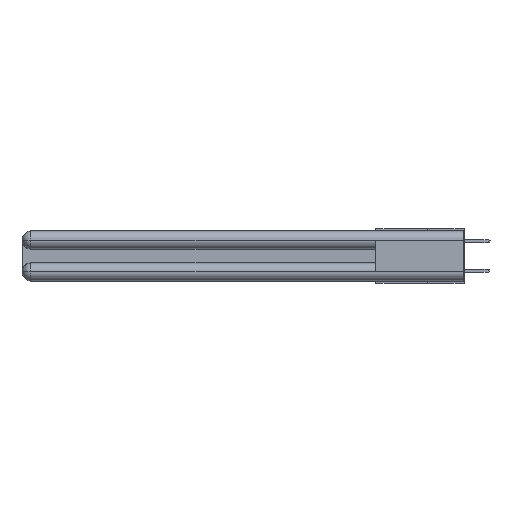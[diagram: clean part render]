
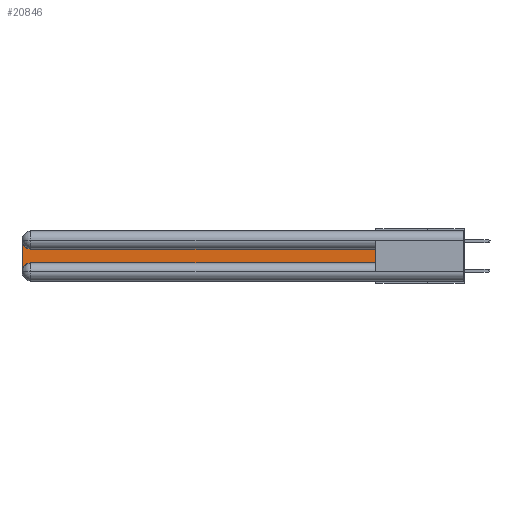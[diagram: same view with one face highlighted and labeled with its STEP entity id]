
A CAD part, left-side view. The second image highlights one B-rep face of the part: STEP entity #20846.
In plain terms, the highlighted planar face has unit normal (-1, 0, 0).
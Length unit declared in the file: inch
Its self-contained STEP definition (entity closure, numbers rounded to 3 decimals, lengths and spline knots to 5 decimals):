
#2008 = FACE_OUTER_BOUND ( 'NONE', #24947, .T. ) ;
#2785 = AXIS2_PLACEMENT_3D ( 'NONE', #3034, #21613, #30291 ) ;
#3034 = CARTESIAN_POINT ( 'NONE',  ( 0.075, 3., -0.1225 ) ) ;
#3149 = PLANE ( 'NONE',  #2785 ) ;
#3286 = EDGE_CURVE ( 'NONE', #6615, #20728, #32143, .T. ) ;
#3447 = VERTEX_POINT ( 'NONE', #4964 ) ;
#3922 = EDGE_CURVE ( 'NONE', #20071, #6615, #4162, .T. ) ;
#4162 = LINE ( 'NONE', #4510, #31746 ) ;
#4510 = CARTESIAN_POINT ( 'NONE',  ( 0.075, 3., -0.2175 ) ) ;
#4614 = DIRECTION ( 'NONE',  ( 0., 0., -1. ) ) ;
#4964 = CARTESIAN_POINT ( 'NONE',  ( 0.075, 0.6, -0.2175 ) ) ;
#6251 = EDGE_CURVE ( 'NONE', #20728, #3447, #19456, .T. ) ;
#6615 = VERTEX_POINT ( 'NONE', #19800 ) ;
#10061 = VERTEX_POINT ( 'NONE', #17948 ) ;
#10757 = VECTOR ( 'NONE', #32738, 39.37008 ) ;
#11026 = CARTESIAN_POINT ( 'NONE',  ( 0.075, 2.94, -0.0625 ) ) ;
#11785 = ORIENTED_EDGE ( 'NONE', *, *, #22195, .T. ) ;
#11967 = EDGE_CURVE ( 'NONE', #10061, #21042, #24591, .T. ) ;
#12924 = DIRECTION ( 'NONE',  ( 0., -1., 0. ) ) ;
#13314 = VECTOR ( 'NONE', #24391, 39.37008 ) ;
#14366 = ORIENTED_EDGE ( 'NONE', *, *, #6251, .T. ) ;
#14448 = CARTESIAN_POINT ( 'NONE',  ( 0.075, 2.94, -0.2775 ) ) ;
#15143 = CARTESIAN_POINT ( 'NONE',  ( 0.075, 0.6, -0.2175 ) ) ;
#16503 = CARTESIAN_POINT ( 'NONE',  ( 0.075, 0.6, -0.2175 ) ) ;
#17138 = DIRECTION ( 'NONE',  ( 0., 0., -1. ) ) ;
#17257 = EDGE_CURVE ( 'NONE', #3447, #10061, #17400, .T. ) ;
#17400 = LINE ( 'NONE', #16503, #10757 ) ;
#17948 = CARTESIAN_POINT ( 'NONE',  ( 0.075, 0.6, -0.1225 ) ) ;
#19186 = CARTESIAN_POINT ( 'NONE',  ( 0.075, 2.94, -0.2175 ) ) ;
#19456 = LINE ( 'NONE', #15143, #27365 ) ;
#19800 = CARTESIAN_POINT ( 'NONE',  ( 0.075, 3., -0.2775 ) ) ;
#20071 = VERTEX_POINT ( 'NONE', #20740 ) ;
#20553 = ORIENTED_EDGE ( 'NONE', *, *, #11967, .T. ) ;
#20728 = VERTEX_POINT ( 'NONE', #19186 ) ;
#20740 = CARTESIAN_POINT ( 'NONE',  ( 0.075, 3., -0.0625 ) ) ;
#20846 = ADVANCED_FACE ( 'NONE', ( #2008 ), #3149, .F. ) ;
#21042 = VERTEX_POINT ( 'NONE', #28380 ) ;
#21613 = DIRECTION ( 'NONE',  ( 1., 0., 0. ) ) ;
#22195 = EDGE_CURVE ( 'NONE', #21042, #20071, #31600, .T. ) ;
#22766 = ORIENTED_EDGE ( 'NONE', *, *, #17257, .T. ) ;
#23244 = ORIENTED_EDGE ( 'NONE', *, *, #3922, .T. ) ;
#24116 = ORIENTED_EDGE ( 'NONE', *, *, #3286, .T. ) ;
#24391 = DIRECTION ( 'NONE',  ( 0., 1., 0. ) ) ;
#24591 = LINE ( 'NONE', #26963, #13314 ) ;
#24947 = EDGE_LOOP ( 'NONE', ( #20553, #11785, #23244, #24116, #14366, #22766 ) ) ;
#26963 = CARTESIAN_POINT ( 'NONE',  ( 0.075, 0.6, -0.1225 ) ) ;
#27222 = DIRECTION ( 'NONE',  ( 1., 0., 0. ) ) ;
#27365 = VECTOR ( 'NONE', #12924, 39.37008 ) ;
#28380 = CARTESIAN_POINT ( 'NONE',  ( 0.075, 2.94, -0.1225 ) ) ;
#30291 = DIRECTION ( 'NONE',  ( 0., 0., -1. ) ) ;
#30498 = AXIS2_PLACEMENT_3D ( 'NONE', #14448, #33152, #17138 ) ;
#31600 = CIRCLE ( 'NONE', #34391, 0.06 ) ;
#31746 = VECTOR ( 'NONE', #4614, 39.37008 ) ;
#32143 = CIRCLE ( 'NONE', #30498, 0.06 ) ;
#32272 = DIRECTION ( 'NONE',  ( 0., 0., -1. ) ) ;
#32738 = DIRECTION ( 'NONE',  ( 0., 0., 1. ) ) ;
#33152 = DIRECTION ( 'NONE',  ( 1., 0., 0. ) ) ;
#34391 = AXIS2_PLACEMENT_3D ( 'NONE', #11026, #27222, #32272 ) ;
